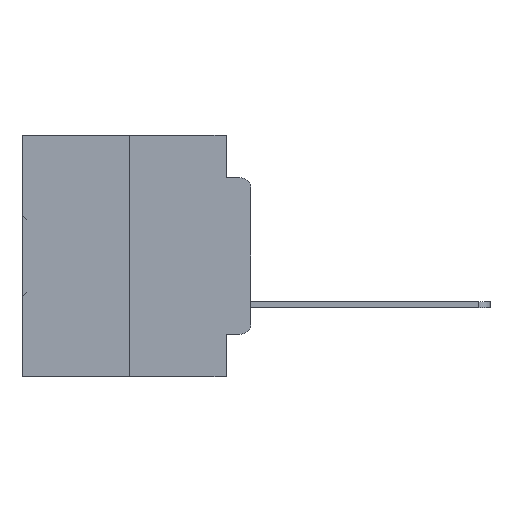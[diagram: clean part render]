
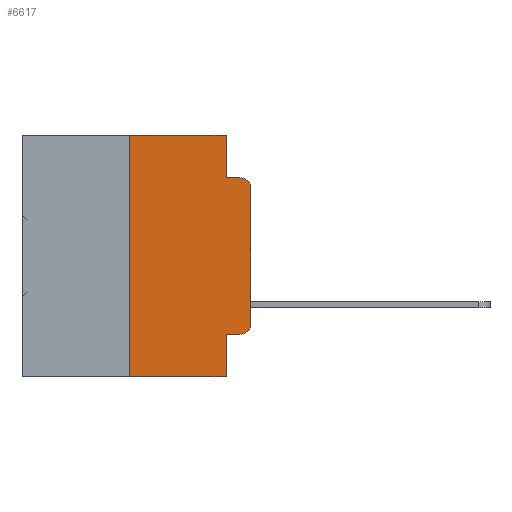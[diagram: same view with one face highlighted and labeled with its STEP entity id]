
A CAD part, left-side view. The second image highlights one B-rep face of the part: STEP entity #6617.
In plain terms, the highlighted planar face has unit normal (-1, 0, 0).
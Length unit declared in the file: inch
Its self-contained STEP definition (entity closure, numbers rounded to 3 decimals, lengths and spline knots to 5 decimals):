
#198 = LINE ( 'NONE', #16960, #29534 ) ;
#701 = CARTESIAN_POINT ( 'NONE',  ( 0., 0.02, -0.3915 ) ) ;
#1377 = AXIS2_PLACEMENT_3D ( 'NONE', #25974, #9095, #28719 ) ;
#1378 = VECTOR ( 'NONE', #17344, 39.37008 ) ;
#1518 = VECTOR ( 'NONE', #26655, 39.37008 ) ;
#1884 = LINE ( 'NONE', #8315, #24616 ) ;
#3030 = DIRECTION ( 'NONE',  ( 0., -1., 0. ) ) ;
#3266 = ORIENTED_EDGE ( 'NONE', *, *, #23578, .T. ) ;
#3662 = DIRECTION ( 'NONE',  ( 0., 0., -1. ) ) ;
#4134 = CARTESIAN_POINT ( 'NONE',  ( 0., 0.02, -0.4115 ) ) ;
#4786 = AXIS2_PLACEMENT_3D ( 'NONE', #11624, #14464, #33931 ) ;
#4844 = AXIS2_PLACEMENT_3D ( 'NONE', #701, #20788, #3662 ) ;
#5068 = EDGE_LOOP ( 'NONE', ( #3266, #5099, #5877, #6449, #7468, #11775, #13577, #15580, #16016, #17354 ) ) ;
#5099 = ORIENTED_EDGE ( 'NONE', *, *, #19865, .T. ) ;
#5343 = EDGE_CURVE ( 'NONE', #33129, #24275, #25037, .T. ) ;
#5877 = ORIENTED_EDGE ( 'NONE', *, *, #12240, .F. ) ;
#6093 = CIRCLE ( 'NONE', #4844, 0.02 ) ;
#6449 = ORIENTED_EDGE ( 'NONE', *, *, #8508, .F. ) ;
#6617 = ADVANCED_FACE ( 'NONE', ( #25821 ), #33822, .F. ) ;
#6925 = LINE ( 'NONE', #34667, #34910 ) ;
#7468 = ORIENTED_EDGE ( 'NONE', *, *, #5343, .F. ) ;
#8315 = CARTESIAN_POINT ( 'NONE',  ( 0., 0.25, 0. ) ) ;
#8508 = EDGE_CURVE ( 'NONE', #24275, #18568, #198, .T. ) ;
#9095 = DIRECTION ( 'NONE',  ( -1., 0., 0. ) ) ;
#9644 = DIRECTION ( 'NONE',  ( 0., -1., 0. ) ) ;
#9647 = CARTESIAN_POINT ( 'NONE',  ( 0., 0.051, -0.0885 ) ) ;
#9941 = LINE ( 'NONE', #11733, #22336 ) ;
#10659 = LINE ( 'NONE', #14587, #17367 ) ;
#10803 = VERTEX_POINT ( 'NONE', #30459 ) ;
#11624 = CARTESIAN_POINT ( 'NONE',  ( 0., 0.473, 0. ) ) ;
#11733 = CARTESIAN_POINT ( 'NONE',  ( 0., 0.473, -0.5 ) ) ;
#11775 = ORIENTED_EDGE ( 'NONE', *, *, #29831, .F. ) ;
#12240 = EDGE_CURVE ( 'NONE', #18568, #10803, #16856, .T. ) ;
#13577 = ORIENTED_EDGE ( 'NONE', *, *, #36564, .T. ) ;
#13677 = VERTEX_POINT ( 'NONE', #29061 ) ;
#14464 = DIRECTION ( 'NONE',  ( 1., 0., 0. ) ) ;
#14587 = CARTESIAN_POINT ( 'NONE',  ( 0., 0.051, 0. ) ) ;
#15315 = CARTESIAN_POINT ( 'NONE',  ( 0., 0., -0.3915 ) ) ;
#15580 = ORIENTED_EDGE ( 'NONE', *, *, #33267, .F. ) ;
#16016 = ORIENTED_EDGE ( 'NONE', *, *, #32770, .T. ) ;
#16628 = VERTEX_POINT ( 'NONE', #15315 ) ;
#16856 = LINE ( 'NONE', #9647, #1518 ) ;
#16960 = CARTESIAN_POINT ( 'NONE',  ( 0., 0.051, 0. ) ) ;
#17149 = CARTESIAN_POINT ( 'NONE',  ( 0., 0.051, -0.0885 ) ) ;
#17344 = DIRECTION ( 'NONE',  ( 0., -1., 0. ) ) ;
#17354 = ORIENTED_EDGE ( 'NONE', *, *, #29098, .T. ) ;
#17367 = VECTOR ( 'NONE', #17499, 39.37008 ) ;
#17440 = VERTEX_POINT ( 'NONE', #32782 ) ;
#17499 = DIRECTION ( 'NONE',  ( 0., 0., -1. ) ) ;
#18319 = VECTOR ( 'NONE', #36029, 39.37008 ) ;
#18568 = VERTEX_POINT ( 'NONE', #17149 ) ;
#19502 = CARTESIAN_POINT ( 'NONE',  ( 0., 0., 0. ) ) ;
#19658 = CARTESIAN_POINT ( 'NONE',  ( 0., 0.051, -0.5 ) ) ;
#19865 = EDGE_CURVE ( 'NONE', #19915, #10803, #29610, .T. ) ;
#19915 = VERTEX_POINT ( 'NONE', #34224 ) ;
#20788 = DIRECTION ( 'NONE',  ( -1., 0., 0. ) ) ;
#22336 = VECTOR ( 'NONE', #3030, 39.37008 ) ;
#22982 = CARTESIAN_POINT ( 'NONE',  ( 0., 0.051, 0. ) ) ;
#23578 = EDGE_CURVE ( 'NONE', #16628, #19915, #26628, .T. ) ;
#24275 = VERTEX_POINT ( 'NONE', #22982 ) ;
#24616 = VECTOR ( 'NONE', #30579, 39.37008 ) ;
#25037 = LINE ( 'NONE', #31249, #1378 ) ;
#25821 = FACE_OUTER_BOUND ( 'NONE', #5068, .T. ) ;
#25974 = CARTESIAN_POINT ( 'NONE',  ( 0., 0.02, -0.1085 ) ) ;
#26628 = LINE ( 'NONE', #19502, #18319 ) ;
#26655 = DIRECTION ( 'NONE',  ( 0., -1., 0. ) ) ;
#27493 = VERTEX_POINT ( 'NONE', #19658 ) ;
#28719 = DIRECTION ( 'NONE',  ( 0., 0., -1. ) ) ;
#29061 = CARTESIAN_POINT ( 'NONE',  ( 0., 0.051, -0.4115 ) ) ;
#29098 = EDGE_CURVE ( 'NONE', #33493, #16628, #6093, .T. ) ;
#29534 = VECTOR ( 'NONE', #30901, 39.37008 ) ;
#29610 = CIRCLE ( 'NONE', #1377, 0.02 ) ;
#29831 = EDGE_CURVE ( 'NONE', #17440, #33129, #1884, .T. ) ;
#30459 = CARTESIAN_POINT ( 'NONE',  ( 0., 0.02, -0.0885 ) ) ;
#30579 = DIRECTION ( 'NONE',  ( 0., 0., 1. ) ) ;
#30901 = DIRECTION ( 'NONE',  ( 0., 0., -1. ) ) ;
#31249 = CARTESIAN_POINT ( 'NONE',  ( 0., 0.473, 0. ) ) ;
#32770 = EDGE_CURVE ( 'NONE', #13677, #33493, #6925, .T. ) ;
#32782 = CARTESIAN_POINT ( 'NONE',  ( 0., 0.25, -0.5 ) ) ;
#33129 = VERTEX_POINT ( 'NONE', #33352 ) ;
#33267 = EDGE_CURVE ( 'NONE', #13677, #27493, #10659, .T. ) ;
#33352 = CARTESIAN_POINT ( 'NONE',  ( 0., 0.25, 0. ) ) ;
#33493 = VERTEX_POINT ( 'NONE', #4134 ) ;
#33822 = PLANE ( 'NONE',  #4786 ) ;
#33931 = DIRECTION ( 'NONE',  ( 0., 0., -1. ) ) ;
#34224 = CARTESIAN_POINT ( 'NONE',  ( 0., 0., -0.1085 ) ) ;
#34667 = CARTESIAN_POINT ( 'NONE',  ( 0., 0.051, -0.4115 ) ) ;
#34910 = VECTOR ( 'NONE', #9644, 39.37008 ) ;
#36029 = DIRECTION ( 'NONE',  ( 0., 0., 1. ) ) ;
#36564 = EDGE_CURVE ( 'NONE', #17440, #27493, #9941, .T. ) ;
